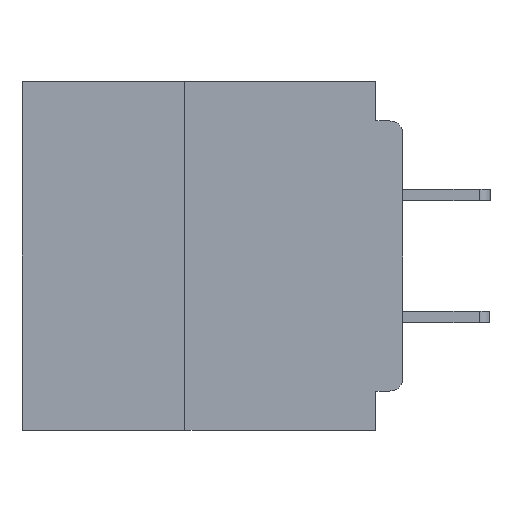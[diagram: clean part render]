
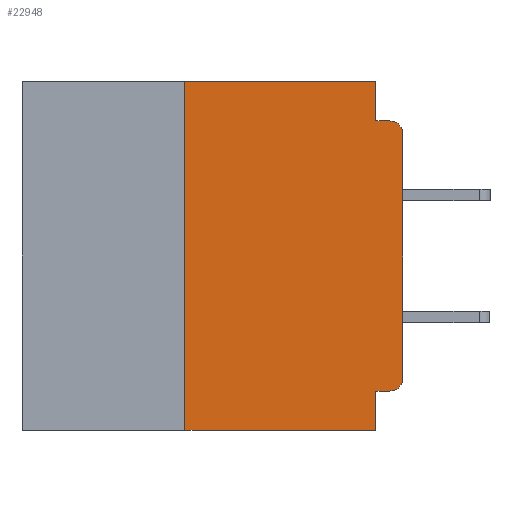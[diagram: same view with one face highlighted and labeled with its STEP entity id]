
A CAD part, left-side view. The second image highlights one B-rep face of the part: STEP entity #22948.
In plain terms, the highlighted planar face has unit normal (-1, 0, 0).
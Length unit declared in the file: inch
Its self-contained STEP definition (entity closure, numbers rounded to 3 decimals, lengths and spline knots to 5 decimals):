
#804 = VERTEX_POINT ( 'NONE', #3098 ) ;
#844 = VECTOR ( 'NONE', #51824, 39.37008 ) ;
#2555 = DIRECTION ( 'NONE',  ( 0., -1., 0. ) ) ;
#3098 = CARTESIAN_POINT ( 'NONE',  ( 0., 0.031, -0.045 ) ) ;
#3541 = ORIENTED_EDGE ( 'NONE', *, *, #44118, .F. ) ;
#3616 = CARTESIAN_POINT ( 'NONE',  ( 0., 0.25, -0.4 ) ) ;
#3868 = ORIENTED_EDGE ( 'NONE', *, *, #45407, .F. ) ;
#3922 = CARTESIAN_POINT ( 'NONE',  ( 0., 0.25, -0.4 ) ) ;
#4344 = CARTESIAN_POINT ( 'NONE',  ( 0., 0., -0.355 ) ) ;
#4975 = CARTESIAN_POINT ( 'NONE',  ( 0., 0.015, -0.34 ) ) ;
#5649 = LINE ( 'NONE', #19537, #15543 ) ;
#6155 = ORIENTED_EDGE ( 'NONE', *, *, #33055, .T. ) ;
#6720 = CARTESIAN_POINT ( 'NONE',  ( 0., 0., -0.045 ) ) ;
#7080 = LINE ( 'NONE', #6720, #50322 ) ;
#7401 = ORIENTED_EDGE ( 'NONE', *, *, #15030, .T. ) ;
#7484 = CARTESIAN_POINT ( 'NONE',  ( 0., 0.031, 0. ) ) ;
#7919 = CARTESIAN_POINT ( 'NONE',  ( 0., 0., 0. ) ) ;
#8542 = DIRECTION ( 'NONE',  ( 0., 1., 0. ) ) ;
#8605 = DIRECTION ( 'NONE',  ( 0., 0., -1. ) ) ;
#9176 = DIRECTION ( 'NONE',  ( 0., 0., -1. ) ) ;
#10075 = DIRECTION ( 'NONE',  ( 0., -1., 0. ) ) ;
#10314 = VERTEX_POINT ( 'NONE', #44011 ) ;
#10327 = ORIENTED_EDGE ( 'NONE', *, *, #20917, .T. ) ;
#10620 = LINE ( 'NONE', #22689, #844 ) ;
#10973 = CIRCLE ( 'NONE', #37303, 0.015 ) ;
#11749 = VECTOR ( 'NONE', #10075, 39.37008 ) ;
#14249 = LINE ( 'NONE', #14398, #45126 ) ;
#14398 = CARTESIAN_POINT ( 'NONE',  ( 0., 0.031, 0. ) ) ;
#14642 = ORIENTED_EDGE ( 'NONE', *, *, #50477, .F. ) ;
#15030 = EDGE_CURVE ( 'NONE', #38596, #38900, #34696, .T. ) ;
#15543 = VECTOR ( 'NONE', #40467, 39.37008 ) ;
#15595 = CARTESIAN_POINT ( 'NONE',  ( 0., 0.015, -0.06 ) ) ;
#17283 = EDGE_CURVE ( 'NONE', #30089, #10314, #10620, .T. ) ;
#17880 = PLANE ( 'NONE',  #29948 ) ;
#18065 = CARTESIAN_POINT ( 'NONE',  ( 0., 0.437, 0. ) ) ;
#18739 = ORIENTED_EDGE ( 'NONE', *, *, #27559, .F. ) ;
#19537 = CARTESIAN_POINT ( 'NONE',  ( 0., 0.437, -0.4 ) ) ;
#19854 = DIRECTION ( 'NONE',  ( 0., 0., -1. ) ) ;
#20917 = EDGE_CURVE ( 'NONE', #28494, #28667, #10973, .T. ) ;
#22316 = DIRECTION ( 'NONE',  ( 0., 0., -1. ) ) ;
#22689 = CARTESIAN_POINT ( 'NONE',  ( 0., 0.031, -0.4 ) ) ;
#22948 = ADVANCED_FACE ( 'NONE', ( #48341 ), #17880, .F. ) ;
#25188 = EDGE_LOOP ( 'NONE', ( #6155, #7401, #50512, #3868, #3541, #18739, #28810, #41255, #14642, #10327 ) ) ;
#26050 = VERTEX_POINT ( 'NONE', #27050 ) ;
#26886 = VECTOR ( 'NONE', #29111, 39.37008 ) ;
#27044 = CARTESIAN_POINT ( 'NONE',  ( 0., 0.437, 0. ) ) ;
#27050 = CARTESIAN_POINT ( 'NONE',  ( 0., 0.25, 0. ) ) ;
#27559 = EDGE_CURVE ( 'NONE', #36391, #26050, #39387, .T. ) ;
#28494 = VERTEX_POINT ( 'NONE', #40460 ) ;
#28667 = VERTEX_POINT ( 'NONE', #41522 ) ;
#28810 = ORIENTED_EDGE ( 'NONE', *, *, #49663, .T. ) ;
#28950 = VECTOR ( 'NONE', #37409, 39.37008 ) ;
#29111 = DIRECTION ( 'NONE',  ( 0., 0., 1. ) ) ;
#29948 = AXIS2_PLACEMENT_3D ( 'NONE', #18065, #47338, #22316 ) ;
#30089 = VERTEX_POINT ( 'NONE', #50734 ) ;
#30585 = LINE ( 'NONE', #4344, #51399 ) ;
#31795 = VERTEX_POINT ( 'NONE', #7484 ) ;
#33055 = EDGE_CURVE ( 'NONE', #28667, #38596, #52389, .T. ) ;
#33929 = AXIS2_PLACEMENT_3D ( 'NONE', #15595, #44964, #19854 ) ;
#34218 = CARTESIAN_POINT ( 'NONE',  ( 0., 0.015, -0.045 ) ) ;
#34358 = EDGE_CURVE ( 'NONE', #804, #38900, #7080, .T. ) ;
#34437 = DIRECTION ( 'NONE',  ( -1., 0., 0. ) ) ;
#34696 = CIRCLE ( 'NONE', #33929, 0.015 ) ;
#35500 = LINE ( 'NONE', #27044, #11749 ) ;
#36391 = VERTEX_POINT ( 'NONE', #3616 ) ;
#37303 = AXIS2_PLACEMENT_3D ( 'NONE', #4975, #34437, #9176 ) ;
#37409 = DIRECTION ( 'NONE',  ( 0., 0., 1. ) ) ;
#38596 = VERTEX_POINT ( 'NONE', #53079 ) ;
#38900 = VERTEX_POINT ( 'NONE', #34218 ) ;
#39387 = LINE ( 'NONE', #3922, #26886 ) ;
#40460 = CARTESIAN_POINT ( 'NONE',  ( 0., 0.015, -0.355 ) ) ;
#40467 = DIRECTION ( 'NONE',  ( 0., -1., 0. ) ) ;
#41255 = ORIENTED_EDGE ( 'NONE', *, *, #17283, .F. ) ;
#41522 = CARTESIAN_POINT ( 'NONE',  ( 0., 0., -0.34 ) ) ;
#44011 = CARTESIAN_POINT ( 'NONE',  ( 0., 0.031, -0.4 ) ) ;
#44118 = EDGE_CURVE ( 'NONE', #26050, #31795, #35500, .T. ) ;
#44964 = DIRECTION ( 'NONE',  ( -1., 0., 0. ) ) ;
#45126 = VECTOR ( 'NONE', #8605, 39.37008 ) ;
#45407 = EDGE_CURVE ( 'NONE', #31795, #804, #14249, .T. ) ;
#47338 = DIRECTION ( 'NONE',  ( 1., 0., 0. ) ) ;
#48341 = FACE_OUTER_BOUND ( 'NONE', #25188, .T. ) ;
#49663 = EDGE_CURVE ( 'NONE', #36391, #10314, #5649, .T. ) ;
#50322 = VECTOR ( 'NONE', #2555, 39.37008 ) ;
#50477 = EDGE_CURVE ( 'NONE', #28494, #30089, #30585, .T. ) ;
#50512 = ORIENTED_EDGE ( 'NONE', *, *, #34358, .F. ) ;
#50734 = CARTESIAN_POINT ( 'NONE',  ( 0., 0.031, -0.355 ) ) ;
#51399 = VECTOR ( 'NONE', #8542, 39.37008 ) ;
#51824 = DIRECTION ( 'NONE',  ( 0., 0., -1. ) ) ;
#52389 = LINE ( 'NONE', #7919, #28950 ) ;
#53079 = CARTESIAN_POINT ( 'NONE',  ( 0., 0., -0.06 ) ) ;
